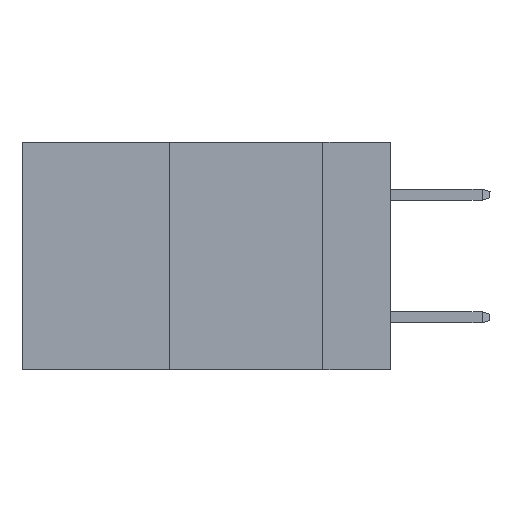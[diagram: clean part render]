
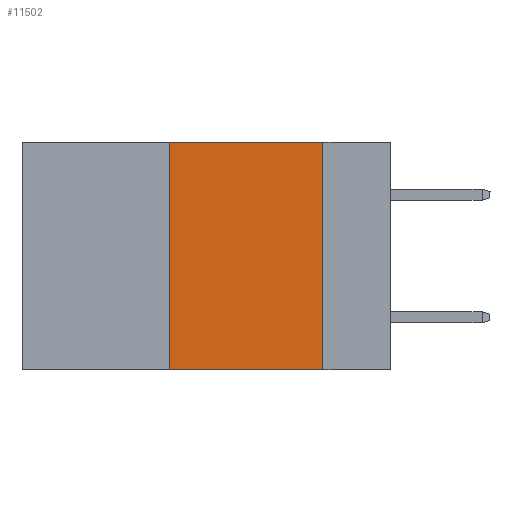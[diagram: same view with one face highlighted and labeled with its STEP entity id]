
A CAD part, left-side view. The second image highlights one B-rep face of the part: STEP entity #11502.
In plain terms, the highlighted planar face has unit normal (-1, 0, 0).
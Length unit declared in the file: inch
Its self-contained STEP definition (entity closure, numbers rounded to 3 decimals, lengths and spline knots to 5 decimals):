
#49 = VERTEX_POINT ( 'NONE', #2111 ) ;
#160 = EDGE_CURVE ( 'NONE', #49, #8528, #4059, .T. ) ;
#369 = VECTOR ( 'NONE', #1554, 39.37008 ) ;
#583 = CARTESIAN_POINT ( 'NONE',  ( 0., 0.6, -0.37 ) ) ;
#746 = VECTOR ( 'NONE', #11525, 39.37008 ) ;
#1405 = EDGE_CURVE ( 'NONE', #11131, #8345, #11264, .T. ) ;
#1554 = DIRECTION ( 'NONE',  ( 0., -1., 0. ) ) ;
#1951 = ORIENTED_EDGE ( 'NONE', *, *, #160, .F. ) ;
#2002 = CARTESIAN_POINT ( 'NONE',  ( 0., 0.11, -0.37 ) ) ;
#2111 = CARTESIAN_POINT ( 'NONE',  ( 0., 0.36, -0.37 ) ) ;
#4059 = LINE ( 'NONE', #6320, #746 ) ;
#4300 = LINE ( 'NONE', #583, #369 ) ;
#4571 = DIRECTION ( 'NONE',  ( 0., -1., 0. ) ) ;
#4671 = VECTOR ( 'NONE', #6360, 39.37008 ) ;
#4677 = EDGE_LOOP ( 'NONE', ( #9051, #4697, #1951, #12290 ) ) ;
#4697 = ORIENTED_EDGE ( 'NONE', *, *, #6834, .F. ) ;
#5187 = VECTOR ( 'NONE', #4571, 39.37008 ) ;
#5226 = EDGE_CURVE ( 'NONE', #49, #8345, #4300, .T. ) ;
#5333 = LINE ( 'NONE', #10572, #5187 ) ;
#5713 = PLANE ( 'NONE',  #6228 ) ;
#6228 = AXIS2_PLACEMENT_3D ( 'NONE', #8047, #9892, #10980 ) ;
#6320 = CARTESIAN_POINT ( 'NONE',  ( 0., 0.36, 0. ) ) ;
#6360 = DIRECTION ( 'NONE',  ( 0., 0., -1. ) ) ;
#6520 = CARTESIAN_POINT ( 'NONE',  ( 0., 0.11, 0. ) ) ;
#6834 = EDGE_CURVE ( 'NONE', #8528, #11131, #5333, .T. ) ;
#8047 = CARTESIAN_POINT ( 'NONE',  ( 0., 0.6, 0. ) ) ;
#8345 = VERTEX_POINT ( 'NONE', #2002 ) ;
#8528 = VERTEX_POINT ( 'NONE', #9643 ) ;
#9051 = ORIENTED_EDGE ( 'NONE', *, *, #1405, .F. ) ;
#9643 = CARTESIAN_POINT ( 'NONE',  ( 0., 0.36, 0. ) ) ;
#9892 = DIRECTION ( 'NONE',  ( 1., 0., 0. ) ) ;
#10415 = FACE_OUTER_BOUND ( 'NONE', #4677, .T. ) ;
#10572 = CARTESIAN_POINT ( 'NONE',  ( 0., 0.6, 0. ) ) ;
#10980 = DIRECTION ( 'NONE',  ( 0., 0., -1. ) ) ;
#11131 = VERTEX_POINT ( 'NONE', #11489 ) ;
#11264 = LINE ( 'NONE', #6520, #4671 ) ;
#11489 = CARTESIAN_POINT ( 'NONE',  ( 0., 0.11, 0. ) ) ;
#11502 = ADVANCED_FACE ( 'NONE', ( #10415 ), #5713, .F. ) ;
#11525 = DIRECTION ( 'NONE',  ( 0., 0., 1. ) ) ;
#12290 = ORIENTED_EDGE ( 'NONE', *, *, #5226, .T. ) ;
